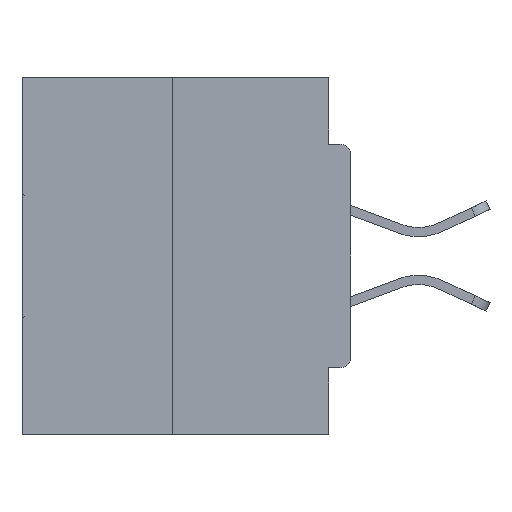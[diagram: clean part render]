
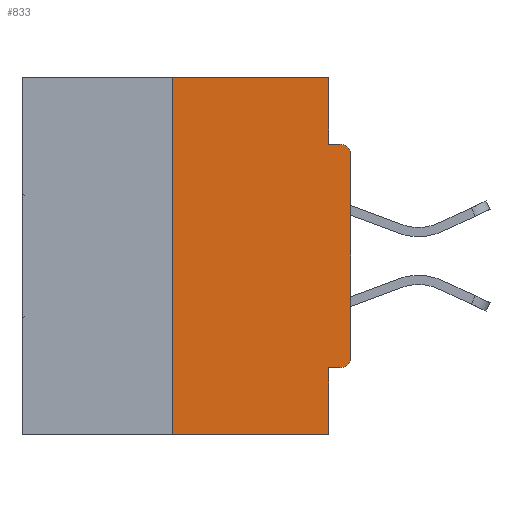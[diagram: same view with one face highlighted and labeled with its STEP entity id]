
A CAD part, left-side view. The second image highlights one B-rep face of the part: STEP entity #833.
In plain terms, the highlighted planar face has unit normal (-1, 0, 0).
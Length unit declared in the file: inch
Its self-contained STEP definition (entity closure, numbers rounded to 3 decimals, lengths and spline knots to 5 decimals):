
#716 = VECTOR ( 'NONE', #23792, 39.37008 ) ;
#833 = ADVANCED_FACE ( 'NONE', ( #1969 ), #7174, .F. ) ;
#842 = DIRECTION ( 'NONE',  ( 0., -1., 0. ) ) ;
#883 = ORIENTED_EDGE ( 'NONE', *, *, #19985, .T. ) ;
#1185 = VECTOR ( 'NONE', #842, 39.37008 ) ;
#1969 = FACE_OUTER_BOUND ( 'NONE', #12910, .T. ) ;
#2619 = CIRCLE ( 'NONE', #17890, 0.015 ) ;
#2839 = CARTESIAN_POINT ( 'NONE',  ( 0., 0., -0.1085 ) ) ;
#3205 = CARTESIAN_POINT ( 'NONE',  ( 0., 0.015, -0.4065 ) ) ;
#3575 = CARTESIAN_POINT ( 'NONE',  ( 0., 0., -0.0935 ) ) ;
#3671 = DIRECTION ( 'NONE',  ( -1., 0., 0. ) ) ;
#3803 = CARTESIAN_POINT ( 'NONE',  ( 0., 0.015, -0.3915 ) ) ;
#4074 = CARTESIAN_POINT ( 'NONE',  ( 0., 0.25, 0. ) ) ;
#4105 = VERTEX_POINT ( 'NONE', #3205 ) ;
#4169 = CARTESIAN_POINT ( 'NONE',  ( 0., 0.46, 0. ) ) ;
#4551 = VERTEX_POINT ( 'NONE', #27098 ) ;
#4628 = ORIENTED_EDGE ( 'NONE', *, *, #20211, .F. ) ;
#4794 = AXIS2_PLACEMENT_3D ( 'NONE', #16211, #3671, #16482 ) ;
#5340 = VERTEX_POINT ( 'NONE', #13546 ) ;
#6474 = VERTEX_POINT ( 'NONE', #7161 ) ;
#6640 = CARTESIAN_POINT ( 'NONE',  ( 0., 0.015, -0.0935 ) ) ;
#7161 = CARTESIAN_POINT ( 'NONE',  ( 0., 0.031, -0.0935 ) ) ;
#7174 = PLANE ( 'NONE',  #19032 ) ;
#7278 = CARTESIAN_POINT ( 'NONE',  ( 0., 0.25, -0.5 ) ) ;
#8482 = EDGE_CURVE ( 'NONE', #32288, #4551, #34459, .T. ) ;
#8486 = ORIENTED_EDGE ( 'NONE', *, *, #11301, .T. ) ;
#8958 = ORIENTED_EDGE ( 'NONE', *, *, #27740, .T. ) ;
#8993 = LINE ( 'NONE', #11817, #716 ) ;
#9438 = EDGE_CURVE ( 'NONE', #14163, #34059, #39770, .T. ) ;
#9663 = VECTOR ( 'NONE', #11142, 39.37008 ) ;
#9748 = VECTOR ( 'NONE', #19475, 39.37008 ) ;
#9942 = LINE ( 'NONE', #3575, #1185 ) ;
#10063 = ORIENTED_EDGE ( 'NONE', *, *, #27137, .F. ) ;
#10601 = DIRECTION ( 'NONE',  ( 0., 0., -1. ) ) ;
#11142 = DIRECTION ( 'NONE',  ( 0., 0., -1. ) ) ;
#11239 = EDGE_CURVE ( 'NONE', #6474, #13262, #9942, .T. ) ;
#11301 = EDGE_CURVE ( 'NONE', #14163, #4551, #12897, .T. ) ;
#11817 = CARTESIAN_POINT ( 'NONE',  ( 0., 0., -0.4065 ) ) ;
#12897 = LINE ( 'NONE', #13003, #35725 ) ;
#12910 = EDGE_LOOP ( 'NONE', ( #10063, #18291, #8486, #13553, #26285, #22337, #883, #8958, #31968, #4628 ) ) ;
#12949 = CARTESIAN_POINT ( 'NONE',  ( 0., 0.031, 0. ) ) ;
#13003 = CARTESIAN_POINT ( 'NONE',  ( 0., 0.46, -0.5 ) ) ;
#13262 = VERTEX_POINT ( 'NONE', #6640 ) ;
#13546 = CARTESIAN_POINT ( 'NONE',  ( 0., 0., -0.3915 ) ) ;
#13553 = ORIENTED_EDGE ( 'NONE', *, *, #8482, .F. ) ;
#14163 = VERTEX_POINT ( 'NONE', #7278 ) ;
#16077 = VECTOR ( 'NONE', #26738, 39.37008 ) ;
#16211 = CARTESIAN_POINT ( 'NONE',  ( 0., 0.015, -0.1085 ) ) ;
#16482 = DIRECTION ( 'NONE',  ( 0., 0., -1. ) ) ;
#16602 = CARTESIAN_POINT ( 'NONE',  ( 0., 0.031, -0.5 ) ) ;
#17509 = EDGE_CURVE ( 'NONE', #4105, #32288, #8993, .T. ) ;
#17807 = EDGE_CURVE ( 'NONE', #4105, #5340, #2619, .T. ) ;
#17890 = AXIS2_PLACEMENT_3D ( 'NONE', #3803, #31820, #10601 ) ;
#18291 = ORIENTED_EDGE ( 'NONE', *, *, #9438, .F. ) ;
#19032 = AXIS2_PLACEMENT_3D ( 'NONE', #4169, #38184, #22683 ) ;
#19475 = DIRECTION ( 'NONE',  ( 0., 0., -1. ) ) ;
#19506 = LINE ( 'NONE', #35691, #16077 ) ;
#19539 = DIRECTION ( 'NONE',  ( 0., -1., 0. ) ) ;
#19985 = EDGE_CURVE ( 'NONE', #5340, #32763, #19506, .T. ) ;
#19996 = LINE ( 'NONE', #12949, #9748 ) ;
#20140 = LINE ( 'NONE', #28738, #36170 ) ;
#20211 = EDGE_CURVE ( 'NONE', #35433, #6474, #19996, .T. ) ;
#22337 = ORIENTED_EDGE ( 'NONE', *, *, #17807, .T. ) ;
#22683 = DIRECTION ( 'NONE',  ( 0., 0., -1. ) ) ;
#23792 = DIRECTION ( 'NONE',  ( 0., 1., 0. ) ) ;
#24184 = VECTOR ( 'NONE', #24908, 39.37008 ) ;
#24908 = DIRECTION ( 'NONE',  ( 0., 0., 1. ) ) ;
#26285 = ORIENTED_EDGE ( 'NONE', *, *, #17509, .F. ) ;
#26738 = DIRECTION ( 'NONE',  ( 0., 0., 1. ) ) ;
#27098 = CARTESIAN_POINT ( 'NONE',  ( 0., 0.031, -0.5 ) ) ;
#27137 = EDGE_CURVE ( 'NONE', #34059, #35433, #20140, .T. ) ;
#27740 = EDGE_CURVE ( 'NONE', #32763, #13262, #38082, .T. ) ;
#28738 = CARTESIAN_POINT ( 'NONE',  ( 0., 0.46, 0. ) ) ;
#30255 = CARTESIAN_POINT ( 'NONE',  ( 0., 0.25, 0. ) ) ;
#31820 = DIRECTION ( 'NONE',  ( -1., 0., 0. ) ) ;
#31968 = ORIENTED_EDGE ( 'NONE', *, *, #11239, .F. ) ;
#32288 = VERTEX_POINT ( 'NONE', #35114 ) ;
#32763 = VERTEX_POINT ( 'NONE', #2839 ) ;
#34059 = VERTEX_POINT ( 'NONE', #30255 ) ;
#34459 = LINE ( 'NONE', #16602, #9663 ) ;
#35114 = CARTESIAN_POINT ( 'NONE',  ( 0., 0.031, -0.4065 ) ) ;
#35433 = VERTEX_POINT ( 'NONE', #39372 ) ;
#35691 = CARTESIAN_POINT ( 'NONE',  ( 0., 0., 0. ) ) ;
#35725 = VECTOR ( 'NONE', #19539, 39.37008 ) ;
#36170 = VECTOR ( 'NONE', #37822, 39.37008 ) ;
#37822 = DIRECTION ( 'NONE',  ( 0., -1., 0. ) ) ;
#38082 = CIRCLE ( 'NONE', #4794, 0.015 ) ;
#38184 = DIRECTION ( 'NONE',  ( 1., 0., 0. ) ) ;
#39372 = CARTESIAN_POINT ( 'NONE',  ( 0., 0.031, 0. ) ) ;
#39770 = LINE ( 'NONE', #4074, #24184 ) ;
